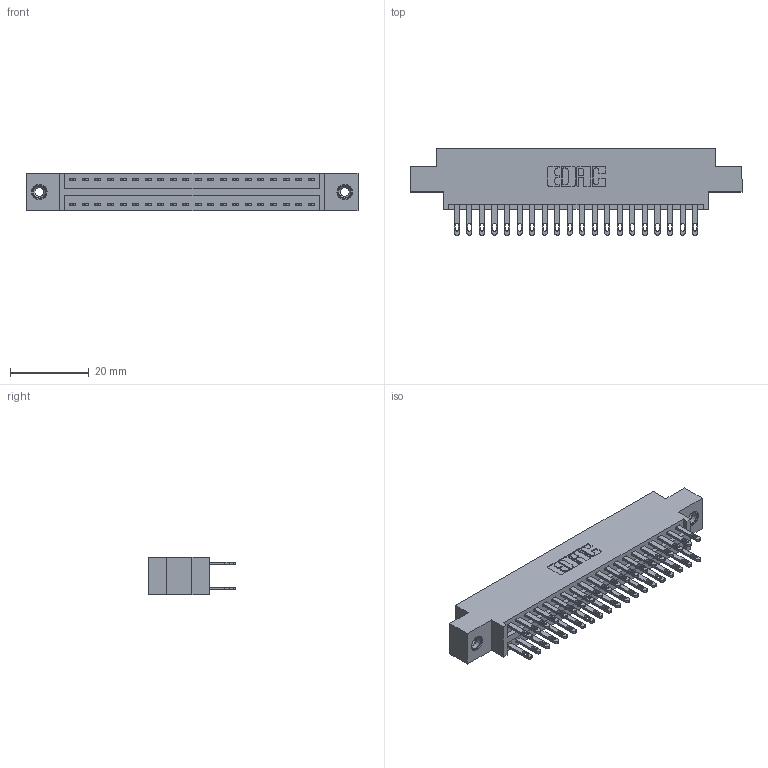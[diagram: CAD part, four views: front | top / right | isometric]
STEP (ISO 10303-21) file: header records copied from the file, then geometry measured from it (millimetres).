
FILE_DESCRIPTION (( 'STEP AP203' ), '1' );
FILE_NAME ('346-040-500-808.STEP', '2022-05-20T01:06:28', ( '' ), ( '' ), 'SwSTEP 2.0', 'SolidWorks 2020', '' );
FILE_SCHEMA (( 'CONFIG_CONTROL_DESIGN' ));
Length unit declared in the file: inch
Products named in the file (4): 345-292-001_345-293-100; 345-250-001_345-250-003-102; 346 Part_0.170 Offset - 0.156 Dia-TI; 346-040-500-808
Assembly tree (43 placements, depth 2):
  346-040-500-808
    346 Part_0.170 Offset - 0.156 Dia-TI
    345-292-001_345-293-100  x40
    345-250-001_345-250-003-102  x2
Bounding box: 84.07 x 21.84 x 9.4 mm (x, y, z)
Volume: 7988.5 mm3; surface area: 11253.2 mm2
Topology: 43 solids, 43 shells, 2106 faces, 6357 edges, 4230 vertices
Faces by surface type: plane 1272, cylinder 818, cone 12, torus 4
Entity records: 17262 total; most frequent: CARTESIAN_POINT 2859, ORIENTED_EDGE 2786, DIRECTION 2599, EDGE_CURVE 1393, VECTOR 1157, LINE 1157, VERTEX_POINT 924, AXIS2_PLACEMENT_3D 721
